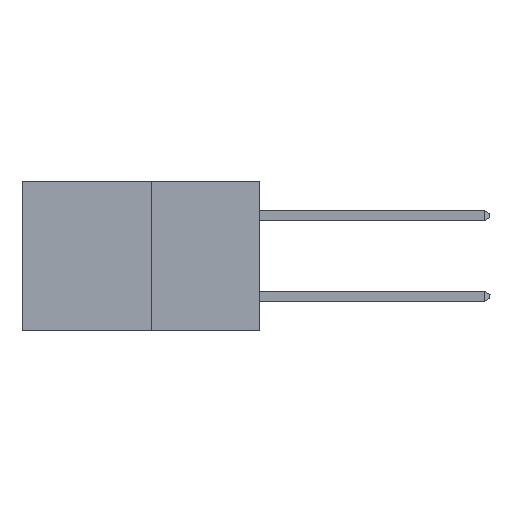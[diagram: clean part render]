
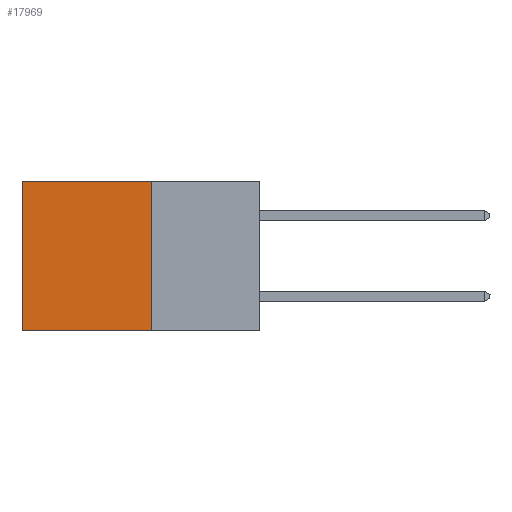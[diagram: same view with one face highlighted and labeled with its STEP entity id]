
A CAD part, left-side view. The second image highlights one B-rep face of the part: STEP entity #17969.
In plain terms, the highlighted planar face has unit normal (-1, 0, 0).
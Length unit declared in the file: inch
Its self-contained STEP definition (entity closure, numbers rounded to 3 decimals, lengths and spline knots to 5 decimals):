
#260 = DIRECTION ( 'NONE',  ( 0., 1., 0. ) ) ;
#495 = EDGE_CURVE ( 'NONE', #14146, #29071, #13163, .T. ) ;
#2327 = LINE ( 'NONE', #32331, #22830 ) ;
#3351 = CARTESIAN_POINT ( 'NONE',  ( 0.277, 0.59, -0.37 ) ) ;
#3923 = VECTOR ( 'NONE', #16325, 39.37008 ) ;
#4767 = LINE ( 'NONE', #18102, #3923 ) ;
#5762 = EDGE_CURVE ( 'NONE', #23587, #14146, #4767, .T. ) ;
#6045 = DIRECTION ( 'NONE',  ( 0., 0., -1. ) ) ;
#7305 = VECTOR ( 'NONE', #6045, 39.37008 ) ;
#10056 = CARTESIAN_POINT ( 'NONE',  ( 0.277, 0.27, -0.37 ) ) ;
#10515 = AXIS2_PLACEMENT_3D ( 'NONE', #10056, #28892, #12865 ) ;
#11659 = CARTESIAN_POINT ( 'NONE',  ( 0.277, 0.59, 0. ) ) ;
#12865 = DIRECTION ( 'NONE',  ( 0., 0., -1. ) ) ;
#13163 = LINE ( 'NONE', #16247, #32763 ) ;
#13471 = FACE_OUTER_BOUND ( 'NONE', #21001, .T. ) ;
#13587 = ORIENTED_EDGE ( 'NONE', *, *, #22548, .F. ) ;
#14146 = VERTEX_POINT ( 'NONE', #11659 ) ;
#16095 = DIRECTION ( 'NONE',  ( 0., 0., -1. ) ) ;
#16247 = CARTESIAN_POINT ( 'NONE',  ( 0.277, 0.59, -0.37 ) ) ;
#16325 = DIRECTION ( 'NONE',  ( 0., 1., 0. ) ) ;
#16706 = CARTESIAN_POINT ( 'NONE',  ( 0.277, 0.27, 0. ) ) ;
#17969 = ADVANCED_FACE ( 'NONE', ( #13471 ), #31413, .F. ) ;
#18102 = CARTESIAN_POINT ( 'NONE',  ( 0.277, 0.27, 0. ) ) ;
#20264 = ORIENTED_EDGE ( 'NONE', *, *, #495, .T. ) ;
#21001 = EDGE_LOOP ( 'NONE', ( #20264, #13587, #27048, #23267 ) ) ;
#22060 = CARTESIAN_POINT ( 'NONE',  ( 0.277, 0.27, -0.37 ) ) ;
#22548 = EDGE_CURVE ( 'NONE', #27120, #29071, #2327, .T. ) ;
#22830 = VECTOR ( 'NONE', #260, 39.37008 ) ;
#23267 = ORIENTED_EDGE ( 'NONE', *, *, #5762, .T. ) ;
#23587 = VERTEX_POINT ( 'NONE', #16706 ) ;
#27048 = ORIENTED_EDGE ( 'NONE', *, *, #34388, .F. ) ;
#27120 = VERTEX_POINT ( 'NONE', #32838 ) ;
#28630 = LINE ( 'NONE', #22060, #7305 ) ;
#28892 = DIRECTION ( 'NONE',  ( 1., 0., 0. ) ) ;
#29071 = VERTEX_POINT ( 'NONE', #3351 ) ;
#31413 = PLANE ( 'NONE',  #10515 ) ;
#32331 = CARTESIAN_POINT ( 'NONE',  ( 0.277, 0.27, -0.37 ) ) ;
#32763 = VECTOR ( 'NONE', #16095, 39.37008 ) ;
#32838 = CARTESIAN_POINT ( 'NONE',  ( 0.277, 0.27, -0.37 ) ) ;
#34388 = EDGE_CURVE ( 'NONE', #23587, #27120, #28630, .T. ) ;
